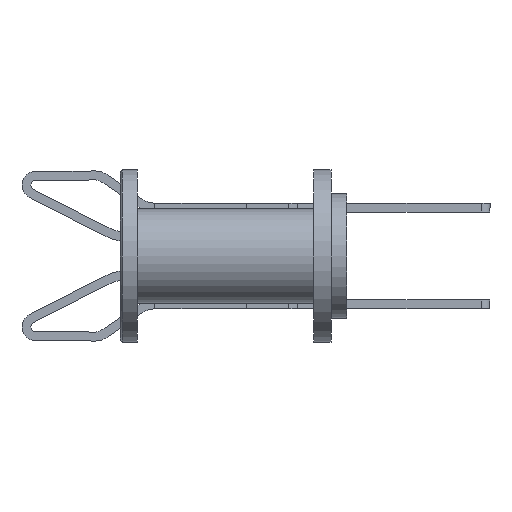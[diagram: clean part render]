
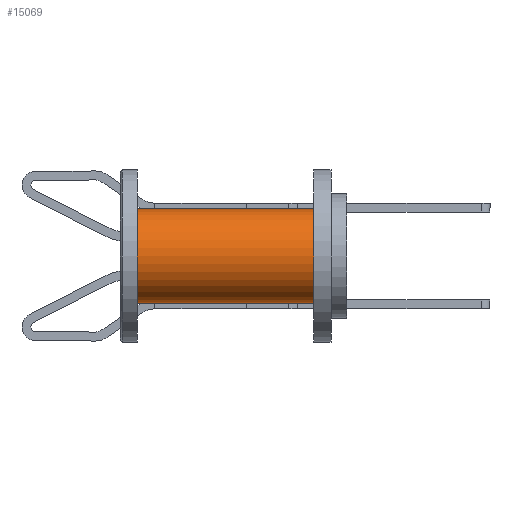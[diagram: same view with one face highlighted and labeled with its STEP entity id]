
A CAD part, left-side view. The second image highlights one B-rep face of the part: STEP entity #15069.
In plain terms, the highlighted cylindrical face has radius 1.727 mm (diameter 3.454 mm), a partial arc.
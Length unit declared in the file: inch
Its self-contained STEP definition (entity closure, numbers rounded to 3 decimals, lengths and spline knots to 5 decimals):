
#1455 = DIRECTION ( 'NONE',  ( 0., -1., 0. ) ) ;
#5119 = ORIENTED_EDGE ( 'NONE', *, *, #34454, .F. ) ;
#6437 = CARTESIAN_POINT ( 'NONE',  ( 0., 0.025, -0.068 ) ) ;
#6640 = DIRECTION ( 'NONE',  ( 0., 1., 0. ) ) ;
#6679 = LINE ( 'NONE', #49665, #48463 ) ;
#10796 = ORIENTED_EDGE ( 'NONE', *, *, #20337, .F. ) ;
#11638 = CARTESIAN_POINT ( 'NONE',  ( 0., 0.328, 0. ) ) ;
#12579 = CARTESIAN_POINT ( 'NONE',  ( 0., 0.28, -0.068 ) ) ;
#14460 = CARTESIAN_POINT ( 'NONE',  ( 0., 0.025, 0.068 ) ) ;
#15069 = ADVANCED_FACE ( 'NONE', ( #22566 ), #53008, .T. ) ;
#15356 = CIRCLE ( 'NONE', #40188, 0.068 ) ;
#15406 = ORIENTED_EDGE ( 'NONE', *, *, #33951, .T. ) ;
#20337 = EDGE_CURVE ( 'NONE', #41358, #49234, #24982, .T. ) ;
#22512 = LINE ( 'NONE', #43248, #32379 ) ;
#22566 = FACE_OUTER_BOUND ( 'NONE', #34225, .T. ) ;
#22837 = ORIENTED_EDGE ( 'NONE', *, *, #39742, .T. ) ;
#24545 = CARTESIAN_POINT ( 'NONE',  ( 0., 0.28, 0. ) ) ;
#24982 = CIRCLE ( 'NONE', #36958, 0.068 ) ;
#28808 = DIRECTION ( 'NONE',  ( 0., 0., 1. ) ) ;
#31890 = CARTESIAN_POINT ( 'NONE',  ( 0., 0.025, 0. ) ) ;
#32379 = VECTOR ( 'NONE', #1455, 39.37008 ) ;
#32392 = VERTEX_POINT ( 'NONE', #6437 ) ;
#32633 = DIRECTION ( 'NONE',  ( 0., 0., -1. ) ) ;
#33951 = EDGE_CURVE ( 'NONE', #52925, #32392, #15356, .T. ) ;
#34225 = EDGE_LOOP ( 'NONE', ( #10796, #22837, #15406, #5119 ) ) ;
#34454 = EDGE_CURVE ( 'NONE', #49234, #32392, #22512, .T. ) ;
#36103 = DIRECTION ( 'NONE',  ( 0., 0., 1. ) ) ;
#36866 = DIRECTION ( 'NONE',  ( 0., -1., 0. ) ) ;
#36958 = AXIS2_PLACEMENT_3D ( 'NONE', #24545, #53468, #28808 ) ;
#39742 = EDGE_CURVE ( 'NONE', #41358, #52925, #6679, .T. ) ;
#39874 = CARTESIAN_POINT ( 'NONE',  ( 0., 0.28, 0.068 ) ) ;
#40188 = AXIS2_PLACEMENT_3D ( 'NONE', #31890, #6640, #36103 ) ;
#41358 = VERTEX_POINT ( 'NONE', #39874 ) ;
#43248 = CARTESIAN_POINT ( 'NONE',  ( 0., 0.328, -0.068 ) ) ;
#43333 = AXIS2_PLACEMENT_3D ( 'NONE', #11638, #36866, #32633 ) ;
#48463 = VECTOR ( 'NONE', #53785, 39.37008 ) ;
#49234 = VERTEX_POINT ( 'NONE', #12579 ) ;
#49665 = CARTESIAN_POINT ( 'NONE',  ( 0., 0.328, 0.068 ) ) ;
#52925 = VERTEX_POINT ( 'NONE', #14460 ) ;
#53008 = CYLINDRICAL_SURFACE ( 'NONE', #43333, 0.068 ) ;
#53468 = DIRECTION ( 'NONE',  ( 0., 1., 0. ) ) ;
#53785 = DIRECTION ( 'NONE',  ( 0., -1., 0. ) ) ;
